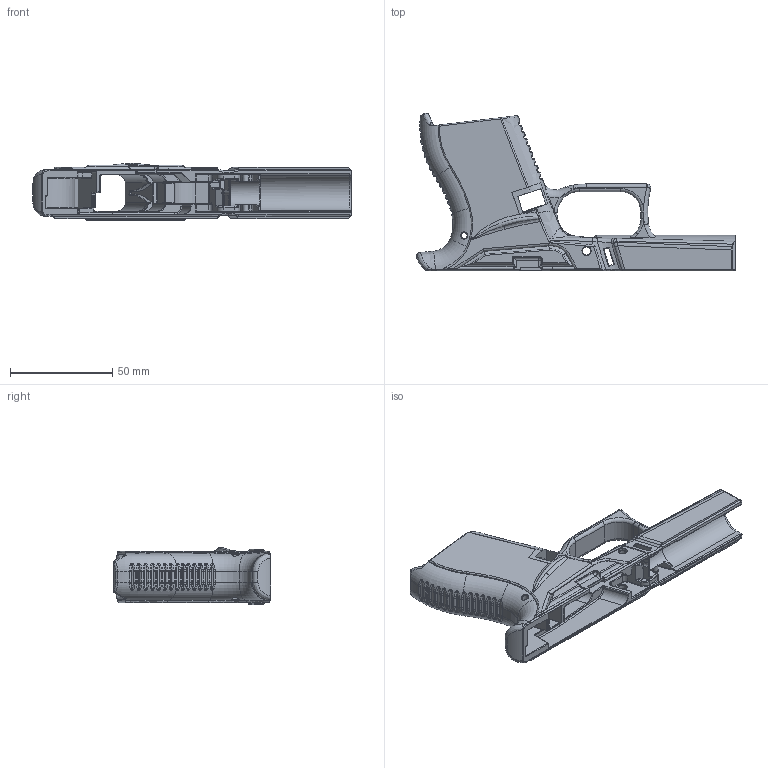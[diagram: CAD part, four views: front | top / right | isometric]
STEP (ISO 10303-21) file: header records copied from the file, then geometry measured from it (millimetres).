
FILE_DESCRIPTION(/* description */ (''),/* implementation_level */ '2;1');
FILE_NAME(/* name */ 'E43v2 v1.step',/* time_stamp */ '2020-07-13T09:56:46-07:00',/* author */ (''),/* organization */ (''),/* preprocessor_version */ 'ST-DEVELOPER v18.1',/* originating_system */ 'Autodesk Translation Framework v9.3.0.1241',/* authorisation */ '');
FILE_SCHEMA (('AUTOMOTIVE_DESIGN { 1 0 10303 214 3 1 1 }'));
Length unit declared in the file: millimetre
Products named in the file (1): E43v2
Bounding box: 155.83 x 77.16 x 27.91 mm (x, y, z)
Volume: 59114.1 mm3; surface area: 32936.3 mm2
Topology: 1 solids, 1 shells, 1312 faces, 3393 edges, 2031 vertices
Faces by surface type: bspline 503, cylinder 421, plane 247, torus 105, sphere 20, cone 16
Full cylindrical faces by diameter (mm): 3 x2, 3.5 x1, 4 x2, 4.5 x2
Entity records: 77048 total; most frequent: CARTESIAN_POINT 48551, ORIENTED_EDGE 6692, DIRECTION 4843, EDGE_CURVE 3346, VERTEX_POINT 2030, AXIS2_PLACEMENT_3D 1869, EDGE_LOOP 1326, FACE_OUTER_BOUND 1311
